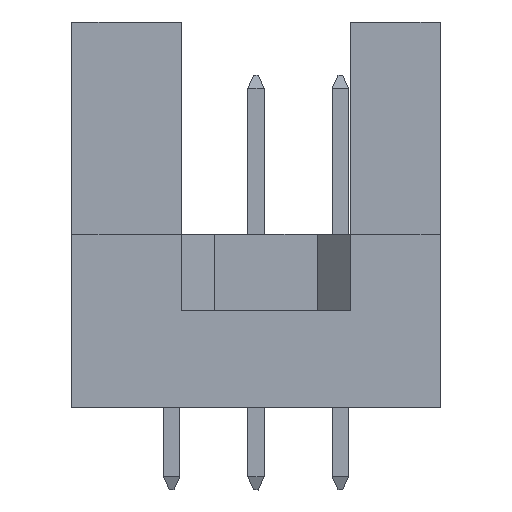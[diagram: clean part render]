
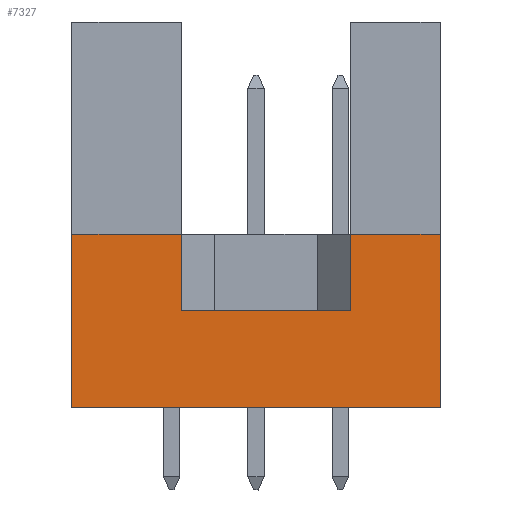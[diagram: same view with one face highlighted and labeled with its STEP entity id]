
A CAD part, left-side view. The second image highlights one B-rep face of the part: STEP entity #7327.
In plain terms, the highlighted planar face has unit normal (-1, 0, 0).
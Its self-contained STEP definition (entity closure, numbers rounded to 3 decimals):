
#45 = VECTOR ( 'NONE', #11411, 1000. ) ;
#102 = VECTOR ( 'NONE', #4011, 1000. ) ;
#130 = VECTOR ( 'NONE', #12059, 1000. ) ;
#240 = DIRECTION ( 'NONE',  ( 0., 0., 1. ) ) ;
#1009 = VERTEX_POINT ( 'NONE', #3590 ) ;
#1870 = EDGE_LOOP ( 'NONE', ( #3061, #3947, #15179, #3408, #15900, #2891, #13219, #16895 ) ) ;
#2116 = VERTEX_POINT ( 'NONE', #15039 ) ;
#2253 = LINE ( 'NONE', #7675, #3014 ) ;
#2891 = ORIENTED_EDGE ( 'NONE', *, *, #7953, .T. ) ;
#2977 = LINE ( 'NONE', #5689, #102 ) ;
#3003 = LINE ( 'NONE', #17024, #45 ) ;
#3014 = VECTOR ( 'NONE', #11980, 1000. ) ;
#3061 = ORIENTED_EDGE ( 'NONE', *, *, #4726, .F. ) ;
#3197 = VERTEX_POINT ( 'NONE', #5894 ) ;
#3408 = ORIENTED_EDGE ( 'NONE', *, *, #16443, .F. ) ;
#3590 = CARTESIAN_POINT ( 'NONE',  ( -47.5, 0., 5.2 ) ) ;
#3683 = EDGE_CURVE ( 'NONE', #14678, #2116, #2977, .T. ) ;
#3917 = VECTOR ( 'NONE', #5604, 1000. ) ;
#3947 = ORIENTED_EDGE ( 'NONE', *, *, #10009, .T. ) ;
#4011 = DIRECTION ( 'NONE',  ( 0., -1., 0. ) ) ;
#4420 = CARTESIAN_POINT ( 'NONE',  ( -47.5, 11.1, 0. ) ) ;
#4726 = EDGE_CURVE ( 'NONE', #3197, #7170, #3003, .T. ) ;
#5008 = EDGE_CURVE ( 'NONE', #5250, #16114, #5680, .T. ) ;
#5198 = CARTESIAN_POINT ( 'NONE',  ( -47.5, 11.1, 0. ) ) ;
#5250 = VERTEX_POINT ( 'NONE', #5198 ) ;
#5604 = DIRECTION ( 'NONE',  ( 0., 0., 1. ) ) ;
#5680 = LINE ( 'NONE', #17174, #6339 ) ;
#5689 = CARTESIAN_POINT ( 'NONE',  ( -47.5, 11.1, 5.2 ) ) ;
#5894 = CARTESIAN_POINT ( 'NONE',  ( -47.5, 7.79, 2.9 ) ) ;
#6074 = LINE ( 'NONE', #14484, #6535 ) ;
#6221 = CARTESIAN_POINT ( 'NONE',  ( -47.5, 7.79, 2.9 ) ) ;
#6339 = VECTOR ( 'NONE', #11380, 1000. ) ;
#6369 = LINE ( 'NONE', #17774, #3917 ) ;
#6535 = VECTOR ( 'NONE', #15797, 1000. ) ;
#7170 = VERTEX_POINT ( 'NONE', #15544 ) ;
#7316 = PLANE ( 'NONE',  #11523 ) ;
#7327 = ADVANCED_FACE ( 'NONE', ( #8628 ), #7316, .F. ) ;
#7400 = VECTOR ( 'NONE', #240, 1000. ) ;
#7675 = CARTESIAN_POINT ( 'NONE',  ( -47.5, 11.1, 0. ) ) ;
#7953 = EDGE_CURVE ( 'NONE', #16114, #1009, #13555, .T. ) ;
#8628 = FACE_OUTER_BOUND ( 'NONE', #1870, .T. ) ;
#8718 = DIRECTION ( 'NONE',  ( 0., 0., -1. ) ) ;
#9515 = CARTESIAN_POINT ( 'NONE',  ( -47.5, 2.71, 5.2 ) ) ;
#10009 = EDGE_CURVE ( 'NONE', #3197, #2116, #11920, .T. ) ;
#10933 = EDGE_CURVE ( 'NONE', #13364, #1009, #6074, .T. ) ;
#11380 = DIRECTION ( 'NONE',  ( 0., -1., 0. ) ) ;
#11411 = DIRECTION ( 'NONE',  ( 0., -1., 0. ) ) ;
#11523 = AXIS2_PLACEMENT_3D ( 'NONE', #4420, #14614, #8718 ) ;
#11920 = LINE ( 'NONE', #6221, #7400 ) ;
#11980 = DIRECTION ( 'NONE',  ( 0., 0., 1. ) ) ;
#12059 = DIRECTION ( 'NONE',  ( 0., 0., 1. ) ) ;
#12461 = CARTESIAN_POINT ( 'NONE',  ( -47.5, 0., 0. ) ) ;
#13219 = ORIENTED_EDGE ( 'NONE', *, *, #10933, .F. ) ;
#13364 = VERTEX_POINT ( 'NONE', #9515 ) ;
#13555 = LINE ( 'NONE', #17680, #130 ) ;
#14484 = CARTESIAN_POINT ( 'NONE',  ( -47.5, 11.1, 5.2 ) ) ;
#14614 = DIRECTION ( 'NONE',  ( 1., 0., 0. ) ) ;
#14678 = VERTEX_POINT ( 'NONE', #15983 ) ;
#15039 = CARTESIAN_POINT ( 'NONE',  ( -47.5, 7.79, 5.2 ) ) ;
#15179 = ORIENTED_EDGE ( 'NONE', *, *, #3683, .F. ) ;
#15544 = CARTESIAN_POINT ( 'NONE',  ( -47.5, 2.71, 2.9 ) ) ;
#15797 = DIRECTION ( 'NONE',  ( 0., -1., 0. ) ) ;
#15900 = ORIENTED_EDGE ( 'NONE', *, *, #5008, .T. ) ;
#15983 = CARTESIAN_POINT ( 'NONE',  ( -47.5, 11.1, 5.2 ) ) ;
#16114 = VERTEX_POINT ( 'NONE', #12461 ) ;
#16443 = EDGE_CURVE ( 'NONE', #5250, #14678, #2253, .T. ) ;
#16460 = EDGE_CURVE ( 'NONE', #7170, #13364, #6369, .T. ) ;
#16895 = ORIENTED_EDGE ( 'NONE', *, *, #16460, .F. ) ;
#17024 = CARTESIAN_POINT ( 'NONE',  ( -47.5, 7.79, 2.9 ) ) ;
#17174 = CARTESIAN_POINT ( 'NONE',  ( -47.5, 11.1, 0. ) ) ;
#17680 = CARTESIAN_POINT ( 'NONE',  ( -47.5, 0., 0. ) ) ;
#17774 = CARTESIAN_POINT ( 'NONE',  ( -47.5, 2.71, 2.9 ) ) ;
